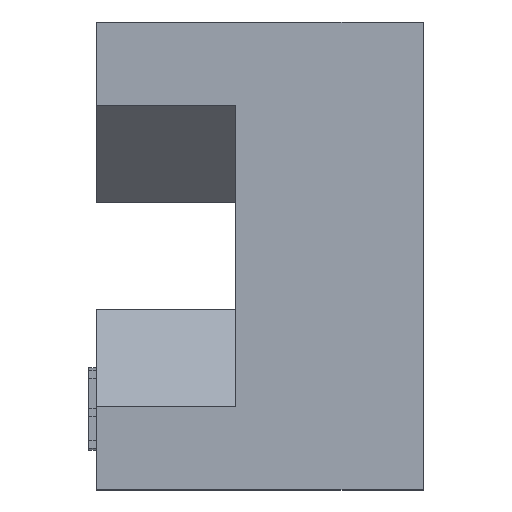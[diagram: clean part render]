
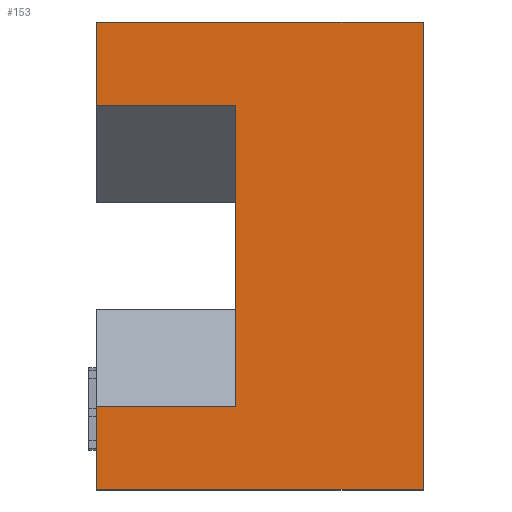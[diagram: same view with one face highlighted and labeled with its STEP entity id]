
A CAD part, left-side view. The second image highlights one B-rep face of the part: STEP entity #153.
In plain terms, the highlighted planar face has unit normal (-1, 0, 0).
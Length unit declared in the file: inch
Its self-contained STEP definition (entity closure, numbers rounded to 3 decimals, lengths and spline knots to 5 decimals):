
#153 = ADVANCED_FACE ( 'NONE', ( #3604 ), #4953, .F. ) ;
#235 = LINE ( 'NONE', #10530, #12370 ) ;
#315 = LINE ( 'NONE', #9564, #682 ) ;
#378 = DIRECTION ( 'NONE',  ( 0., 0., 1. ) ) ;
#682 = VECTOR ( 'NONE', #8295, 39.37008 ) ;
#1231 = EDGE_CURVE ( 'NONE', #8156, #13474, #10433, .T. ) ;
#1464 = CARTESIAN_POINT ( 'NONE',  ( -1.25, 0.218, -0.156 ) ) ;
#1473 = LINE ( 'NONE', #4831, #8534 ) ;
#1551 = CARTESIAN_POINT ( 'NONE',  ( -1.25, 0.125, 0.1005 ) ) ;
#2251 = ORIENTED_EDGE ( 'NONE', *, *, #8311, .T. ) ;
#2332 = VECTOR ( 'NONE', #11240, 39.37008 ) ;
#2400 = LINE ( 'NONE', #7994, #4530 ) ;
#2424 = VERTEX_POINT ( 'NONE', #2591 ) ;
#2508 = CARTESIAN_POINT ( 'NONE',  ( -1.25, 0.218, -0.1005 ) ) ;
#2591 = CARTESIAN_POINT ( 'NONE',  ( -1.25, 0.218, 0.156 ) ) ;
#2602 = DIRECTION ( 'NONE',  ( 0., 1., 0. ) ) ;
#2649 = CARTESIAN_POINT ( 'NONE',  ( -1.25, 0., -0.156 ) ) ;
#2942 = EDGE_CURVE ( 'NONE', #13576, #8156, #4344, .T. ) ;
#3094 = EDGE_CURVE ( 'NONE', #2424, #4968, #6931, .T. ) ;
#3469 = ORIENTED_EDGE ( 'NONE', *, *, #3522, .T. ) ;
#3522 = EDGE_CURVE ( 'NONE', #13576, #10736, #1473, .T. ) ;
#3604 = FACE_OUTER_BOUND ( 'NONE', #9711, .T. ) ;
#3779 = VECTOR ( 'NONE', #11356, 39.37008 ) ;
#3868 = CARTESIAN_POINT ( 'NONE',  ( -1.25, 0., -0.156 ) ) ;
#4224 = AXIS2_PLACEMENT_3D ( 'NONE', #10610, #9352, #6007 ) ;
#4344 = LINE ( 'NONE', #6813, #3779 ) ;
#4530 = VECTOR ( 'NONE', #12628, 39.37008 ) ;
#4831 = CARTESIAN_POINT ( 'NONE',  ( -1.25, 0.125, -0.1005 ) ) ;
#4918 = EDGE_CURVE ( 'NONE', #9494, #10736, #315, .T. ) ;
#4953 = PLANE ( 'NONE',  #4224 ) ;
#4968 = VERTEX_POINT ( 'NONE', #13907 ) ;
#5365 = VERTEX_POINT ( 'NONE', #3868 ) ;
#5860 = LINE ( 'NONE', #2649, #13581 ) ;
#5949 = CARTESIAN_POINT ( 'NONE',  ( -1.25, 0.218, 0.1005 ) ) ;
#6007 = DIRECTION ( 'NONE',  ( 0., 0., -1. ) ) ;
#6440 = EDGE_CURVE ( 'NONE', #13474, #2424, #235, .T. ) ;
#6560 = ORIENTED_EDGE ( 'NONE', *, *, #4918, .F. ) ;
#6813 = CARTESIAN_POINT ( 'NONE',  ( -1.25, 0.125, -0.1005 ) ) ;
#6931 = LINE ( 'NONE', #12519, #2332 ) ;
#6954 = ORIENTED_EDGE ( 'NONE', *, *, #6440, .F. ) ;
#7290 = DIRECTION ( 'NONE',  ( 0., 1., 0. ) ) ;
#7487 = CARTESIAN_POINT ( 'NONE',  ( -1.25, 0.125, 0.1005 ) ) ;
#7994 = CARTESIAN_POINT ( 'NONE',  ( -1.25, 0.218, -0.156 ) ) ;
#8005 = EDGE_CURVE ( 'NONE', #5365, #4968, #5860, .T. ) ;
#8156 = VERTEX_POINT ( 'NONE', #7487 ) ;
#8295 = DIRECTION ( 'NONE',  ( 0., 0., 1. ) ) ;
#8311 = EDGE_CURVE ( 'NONE', #9494, #5365, #2400, .T. ) ;
#8534 = VECTOR ( 'NONE', #7290, 39.37008 ) ;
#8572 = ORIENTED_EDGE ( 'NONE', *, *, #1231, .F. ) ;
#9352 = DIRECTION ( 'NONE',  ( 1., 0., 0. ) ) ;
#9494 = VERTEX_POINT ( 'NONE', #1464 ) ;
#9564 = CARTESIAN_POINT ( 'NONE',  ( -1.25, 0.218, -0.156 ) ) ;
#9711 = EDGE_LOOP ( 'NONE', ( #10159, #3469, #6560, #2251, #11570, #13713, #6954, #8572 ) ) ;
#10159 = ORIENTED_EDGE ( 'NONE', *, *, #2942, .F. ) ;
#10433 = LINE ( 'NONE', #1551, #11887 ) ;
#10530 = CARTESIAN_POINT ( 'NONE',  ( -1.25, 0.218, -0.156 ) ) ;
#10610 = CARTESIAN_POINT ( 'NONE',  ( -1.25, 0.218, -0.156 ) ) ;
#10736 = VERTEX_POINT ( 'NONE', #2508 ) ;
#11240 = DIRECTION ( 'NONE',  ( 0., -1., 0. ) ) ;
#11356 = DIRECTION ( 'NONE',  ( 0., 0., 1. ) ) ;
#11570 = ORIENTED_EDGE ( 'NONE', *, *, #8005, .T. ) ;
#11887 = VECTOR ( 'NONE', #2602, 39.37008 ) ;
#12370 = VECTOR ( 'NONE', #378, 39.37008 ) ;
#12519 = CARTESIAN_POINT ( 'NONE',  ( -1.25, 0.218, 0.156 ) ) ;
#12628 = DIRECTION ( 'NONE',  ( 0., -1., 0. ) ) ;
#13213 = CARTESIAN_POINT ( 'NONE',  ( -1.25, 0.125, -0.1005 ) ) ;
#13474 = VERTEX_POINT ( 'NONE', #5949 ) ;
#13554 = DIRECTION ( 'NONE',  ( 0., 0., 1. ) ) ;
#13576 = VERTEX_POINT ( 'NONE', #13213 ) ;
#13581 = VECTOR ( 'NONE', #13554, 39.37008 ) ;
#13713 = ORIENTED_EDGE ( 'NONE', *, *, #3094, .F. ) ;
#13907 = CARTESIAN_POINT ( 'NONE',  ( -1.25, 0., 0.156 ) ) ;
